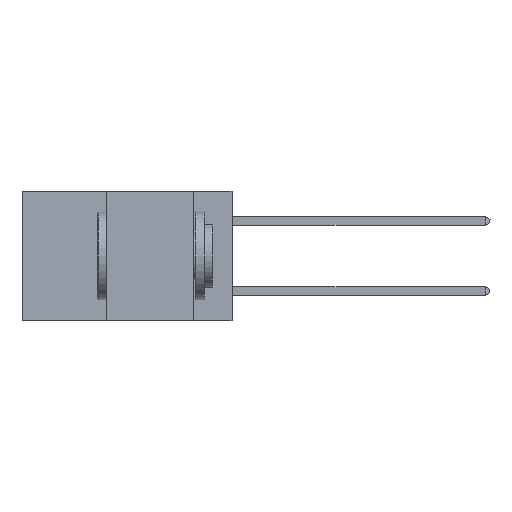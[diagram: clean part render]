
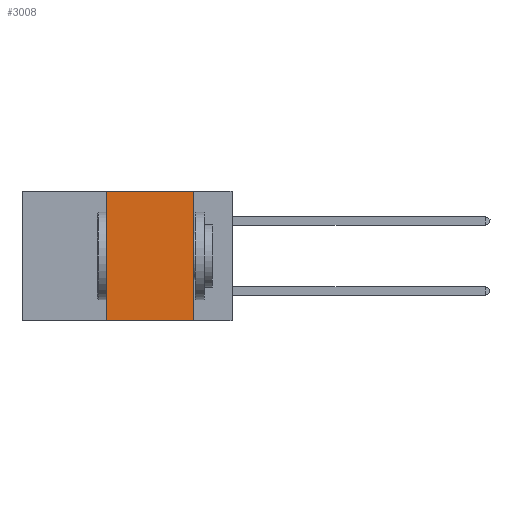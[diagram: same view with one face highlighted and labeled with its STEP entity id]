
A CAD part, left-side view. The second image highlights one B-rep face of the part: STEP entity #3008.
In plain terms, the highlighted planar face has unit normal (-1, 0, 0).
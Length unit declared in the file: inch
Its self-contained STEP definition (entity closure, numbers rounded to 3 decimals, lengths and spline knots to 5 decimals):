
#60 = VERTEX_POINT ( 'NONE', #4608 ) ;
#457 = ORIENTED_EDGE ( 'NONE', *, *, #6924, .F. ) ;
#567 = EDGE_CURVE ( 'NONE', #9124, #1316, #5747, .T. ) ;
#640 = ORIENTED_EDGE ( 'NONE', *, *, #567, .F. ) ;
#673 = CARTESIAN_POINT ( 'NONE',  ( 0., 0.36, 0. ) ) ;
#698 = DIRECTION ( 'NONE',  ( 0., 0., -1. ) ) ;
#1316 = VERTEX_POINT ( 'NONE', #9998 ) ;
#1406 = ORIENTED_EDGE ( 'NONE', *, *, #7275, .F. ) ;
#1526 = CARTESIAN_POINT ( 'NONE',  ( 0., 0.11, 0. ) ) ;
#1543 = LINE ( 'NONE', #673, #2905 ) ;
#1690 = VECTOR ( 'NONE', #9095, 39.37008 ) ;
#2304 = DIRECTION ( 'NONE',  ( 0., 0., -1. ) ) ;
#2905 = VECTOR ( 'NONE', #9917, 39.37008 ) ;
#3008 = ADVANCED_FACE ( 'NONE', ( #6099 ), #9392, .F. ) ;
#3249 = AXIS2_PLACEMENT_3D ( 'NONE', #8506, #4743, #698 ) ;
#3706 = DIRECTION ( 'NONE',  ( 0., -1., 0. ) ) ;
#4608 = CARTESIAN_POINT ( 'NONE',  ( 0., 0.36, 0. ) ) ;
#4743 = DIRECTION ( 'NONE',  ( 1., 0., 0. ) ) ;
#5110 = CARTESIAN_POINT ( 'NONE',  ( 0., 0.36, -0.37 ) ) ;
#5520 = EDGE_CURVE ( 'NONE', #5990, #1316, #8096, .T. ) ;
#5665 = VECTOR ( 'NONE', #3706, 39.37008 ) ;
#5747 = LINE ( 'NONE', #1526, #7062 ) ;
#5990 = VERTEX_POINT ( 'NONE', #5110 ) ;
#6099 = FACE_OUTER_BOUND ( 'NONE', #8955, .T. ) ;
#6144 = CARTESIAN_POINT ( 'NONE',  ( 0., 0.6, 0. ) ) ;
#6924 = EDGE_CURVE ( 'NONE', #60, #9124, #9789, .T. ) ;
#7062 = VECTOR ( 'NONE', #2304, 39.37008 ) ;
#7275 = EDGE_CURVE ( 'NONE', #5990, #60, #1543, .T. ) ;
#7534 = CARTESIAN_POINT ( 'NONE',  ( 0., 0.6, -0.37 ) ) ;
#8096 = LINE ( 'NONE', #7534, #1690 ) ;
#8506 = CARTESIAN_POINT ( 'NONE',  ( 0., 0.6, 0. ) ) ;
#8813 = CARTESIAN_POINT ( 'NONE',  ( 0., 0.11, 0. ) ) ;
#8955 = EDGE_LOOP ( 'NONE', ( #640, #457, #1406, #9914 ) ) ;
#9095 = DIRECTION ( 'NONE',  ( 0., -1., 0. ) ) ;
#9124 = VERTEX_POINT ( 'NONE', #8813 ) ;
#9392 = PLANE ( 'NONE',  #3249 ) ;
#9789 = LINE ( 'NONE', #6144, #5665 ) ;
#9914 = ORIENTED_EDGE ( 'NONE', *, *, #5520, .T. ) ;
#9917 = DIRECTION ( 'NONE',  ( 0., 0., 1. ) ) ;
#9998 = CARTESIAN_POINT ( 'NONE',  ( 0., 0.11, -0.37 ) ) ;
